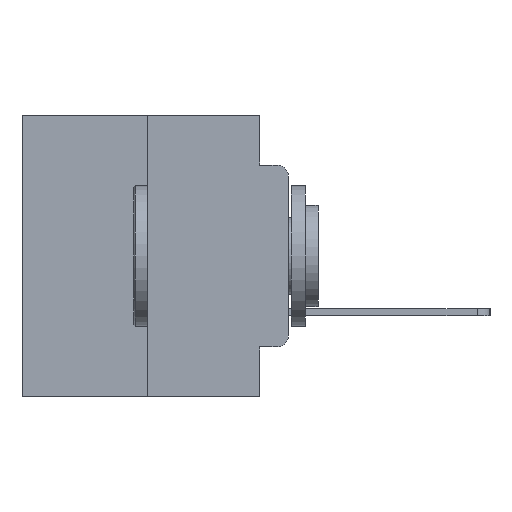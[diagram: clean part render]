
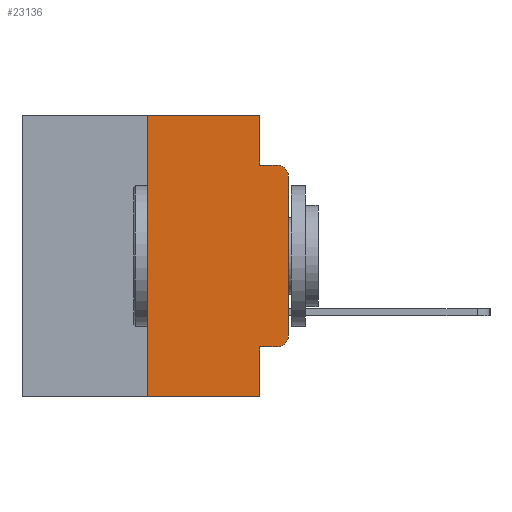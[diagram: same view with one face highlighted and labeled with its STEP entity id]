
A CAD part, left-side view. The second image highlights one B-rep face of the part: STEP entity #23136.
In plain terms, the highlighted planar face has unit normal (-1, 0, 0).
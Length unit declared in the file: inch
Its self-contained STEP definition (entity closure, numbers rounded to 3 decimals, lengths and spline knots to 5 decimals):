
#587 = VECTOR ( 'NONE', #597, 39.37008 ) ;
#597 = DIRECTION ( 'NONE',  ( 0., 0., 1. ) ) ;
#666 = ORIENTED_EDGE ( 'NONE', *, *, #23032, .F. ) ;
#780 = VERTEX_POINT ( 'NONE', #16821 ) ;
#2014 = ORIENTED_EDGE ( 'NONE', *, *, #6119, .T. ) ;
#2238 = LINE ( 'NONE', #18491, #23315 ) ;
#2729 = LINE ( 'NONE', #24399, #19109 ) ;
#3324 = VECTOR ( 'NONE', #8401, 39.37008 ) ;
#3410 = VERTEX_POINT ( 'NONE', #7986 ) ;
#3522 = VECTOR ( 'NONE', #4931, 39.37008 ) ;
#3581 = VERTEX_POINT ( 'NONE', #18530 ) ;
#3759 = EDGE_CURVE ( 'NONE', #3581, #780, #20679, .T. ) ;
#3896 = LINE ( 'NONE', #11147, #8244 ) ;
#4711 = LINE ( 'NONE', #22436, #3324 ) ;
#4929 = DIRECTION ( 'NONE',  ( -1., 0., 0. ) ) ;
#4931 = DIRECTION ( 'NONE',  ( 0., 0., -1. ) ) ;
#5250 = PLANE ( 'NONE',  #15237 ) ;
#5577 = FACE_OUTER_BOUND ( 'NONE', #26522, .T. ) ;
#6083 = ORIENTED_EDGE ( 'NONE', *, *, #14834, .T. ) ;
#6119 = EDGE_CURVE ( 'NONE', #780, #17988, #7657, .T. ) ;
#6167 = VERTEX_POINT ( 'NONE', #21273 ) ;
#6249 = VECTOR ( 'NONE', #11526, 39.37008 ) ;
#6416 = CARTESIAN_POINT ( 'NONE',  ( 0., 0., -0.1085 ) ) ;
#7146 = VERTEX_POINT ( 'NONE', #22204 ) ;
#7657 = LINE ( 'NONE', #13155, #587 ) ;
#7986 = CARTESIAN_POINT ( 'NONE',  ( 0., 0.25, 0. ) ) ;
#8244 = VECTOR ( 'NONE', #25105, 39.37008 ) ;
#8378 = CARTESIAN_POINT ( 'NONE',  ( 0., 0.02, -0.1085 ) ) ;
#8401 = DIRECTION ( 'NONE',  ( 0., 0., 1. ) ) ;
#8957 = CARTESIAN_POINT ( 'NONE',  ( 0., 0.051, -0.0885 ) ) ;
#9526 = CARTESIAN_POINT ( 'NONE',  ( 0., 0.051, -0.4115 ) ) ;
#10405 = CARTESIAN_POINT ( 'NONE',  ( 0., 0.051, -0.4115 ) ) ;
#10426 = DIRECTION ( 'NONE',  ( 0., 0., -1. ) ) ;
#10441 = VERTEX_POINT ( 'NONE', #10405 ) ;
#10551 = DIRECTION ( 'NONE',  ( 0., -1., 0. ) ) ;
#10815 = EDGE_CURVE ( 'NONE', #10441, #3581, #22973, .T. ) ;
#11147 = CARTESIAN_POINT ( 'NONE',  ( 0., 0.473, 0. ) ) ;
#11161 = AXIS2_PLACEMENT_3D ( 'NONE', #17147, #4929, #19141 ) ;
#11526 = DIRECTION ( 'NONE',  ( 0., -1., 0. ) ) ;
#12176 = ORIENTED_EDGE ( 'NONE', *, *, #14850, .F. ) ;
#12429 = DIRECTION ( 'NONE',  ( 0., 0., -1. ) ) ;
#13155 = CARTESIAN_POINT ( 'NONE',  ( 0., 0., 0. ) ) ;
#13521 = DIRECTION ( 'NONE',  ( 0., 0., -1. ) ) ;
#14432 = LINE ( 'NONE', #16298, #19740 ) ;
#14767 = AXIS2_PLACEMENT_3D ( 'NONE', #8378, #22415, #10426 ) ;
#14834 = EDGE_CURVE ( 'NONE', #22322, #7146, #14432, .T. ) ;
#14850 = EDGE_CURVE ( 'NONE', #10441, #7146, #2729, .T. ) ;
#14998 = CARTESIAN_POINT ( 'NONE',  ( 0., 0.051, 0. ) ) ;
#15011 = VERTEX_POINT ( 'NONE', #14998 ) ;
#15237 = AXIS2_PLACEMENT_3D ( 'NONE', #21462, #25442, #13521 ) ;
#16173 = EDGE_CURVE ( 'NONE', #22322, #3410, #4711, .T. ) ;
#16298 = CARTESIAN_POINT ( 'NONE',  ( 0., 0.473, -0.5 ) ) ;
#16585 = ORIENTED_EDGE ( 'NONE', *, *, #10815, .T. ) ;
#16821 = CARTESIAN_POINT ( 'NONE',  ( 0., 0., -0.3915 ) ) ;
#17147 = CARTESIAN_POINT ( 'NONE',  ( 0., 0.02, -0.3915 ) ) ;
#17988 = VERTEX_POINT ( 'NONE', #6416 ) ;
#18491 = CARTESIAN_POINT ( 'NONE',  ( 0., 0.051, -0.0885 ) ) ;
#18530 = CARTESIAN_POINT ( 'NONE',  ( 0., 0.02, -0.4115 ) ) ;
#18737 = ORIENTED_EDGE ( 'NONE', *, *, #20197, .F. ) ;
#19049 = ORIENTED_EDGE ( 'NONE', *, *, #25512, .T. ) ;
#19109 = VECTOR ( 'NONE', #12429, 39.37008 ) ;
#19141 = DIRECTION ( 'NONE',  ( 0., 0., -1. ) ) ;
#19740 = VECTOR ( 'NONE', #20234, 39.37008 ) ;
#19851 = LINE ( 'NONE', #21069, #3522 ) ;
#20197 = EDGE_CURVE ( 'NONE', #15011, #22975, #19851, .T. ) ;
#20234 = DIRECTION ( 'NONE',  ( 0., -1., 0. ) ) ;
#20679 = CIRCLE ( 'NONE', #11161, 0.02 ) ;
#21069 = CARTESIAN_POINT ( 'NONE',  ( 0., 0.051, 0. ) ) ;
#21273 = CARTESIAN_POINT ( 'NONE',  ( 0., 0.02, -0.0885 ) ) ;
#21462 = CARTESIAN_POINT ( 'NONE',  ( 0., 0.473, 0. ) ) ;
#22204 = CARTESIAN_POINT ( 'NONE',  ( 0., 0.051, -0.5 ) ) ;
#22322 = VERTEX_POINT ( 'NONE', #26426 ) ;
#22415 = DIRECTION ( 'NONE',  ( -1., 0., 0. ) ) ;
#22436 = CARTESIAN_POINT ( 'NONE',  ( 0., 0.25, 0. ) ) ;
#22862 = EDGE_CURVE ( 'NONE', #22975, #6167, #2238, .T. ) ;
#22973 = LINE ( 'NONE', #9526, #6249 ) ;
#22975 = VERTEX_POINT ( 'NONE', #8957 ) ;
#23032 = EDGE_CURVE ( 'NONE', #3410, #15011, #3896, .T. ) ;
#23126 = ORIENTED_EDGE ( 'NONE', *, *, #16173, .F. ) ;
#23136 = ADVANCED_FACE ( 'NONE', ( #5577 ), #5250, .F. ) ;
#23147 = ORIENTED_EDGE ( 'NONE', *, *, #3759, .T. ) ;
#23189 = CIRCLE ( 'NONE', #14767, 0.02 ) ;
#23315 = VECTOR ( 'NONE', #10551, 39.37008 ) ;
#23440 = ORIENTED_EDGE ( 'NONE', *, *, #22862, .F. ) ;
#24399 = CARTESIAN_POINT ( 'NONE',  ( 0., 0.051, 0. ) ) ;
#25105 = DIRECTION ( 'NONE',  ( 0., -1., 0. ) ) ;
#25442 = DIRECTION ( 'NONE',  ( 1., 0., 0. ) ) ;
#25512 = EDGE_CURVE ( 'NONE', #17988, #6167, #23189, .T. ) ;
#26426 = CARTESIAN_POINT ( 'NONE',  ( 0., 0.25, -0.5 ) ) ;
#26522 = EDGE_LOOP ( 'NONE', ( #2014, #19049, #23440, #18737, #666, #23126, #6083, #12176, #16585, #23147 ) ) ;
